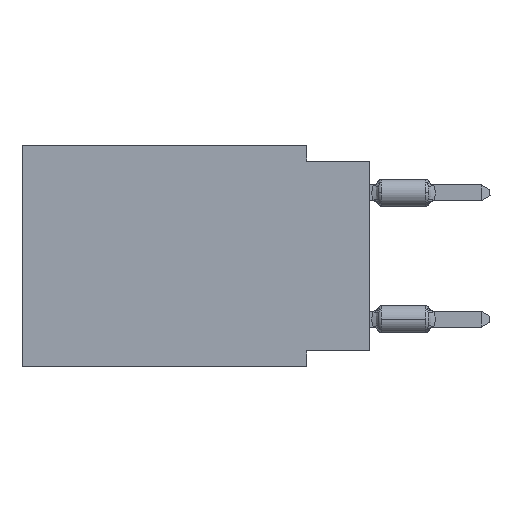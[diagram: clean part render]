
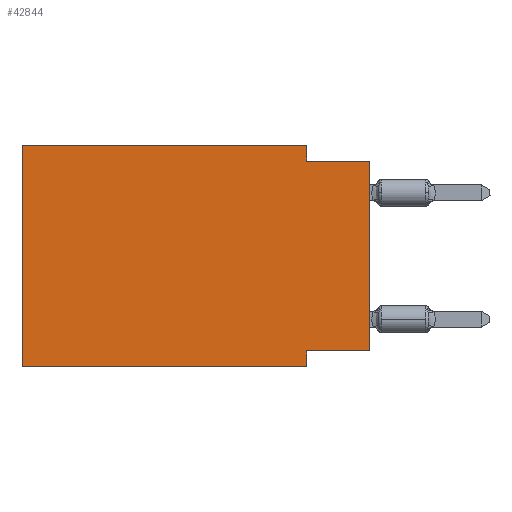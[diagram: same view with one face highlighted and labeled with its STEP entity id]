
A CAD part, left-side view. The second image highlights one B-rep face of the part: STEP entity #42844.
In plain terms, the highlighted planar face has unit normal (-1, 0, 0).
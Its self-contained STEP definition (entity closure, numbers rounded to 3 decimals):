
#47 = LINE ( 'NONE', #48566, #8587 ) ;
#1455 = VERTEX_POINT ( 'NONE', #36097 ) ;
#1940 = EDGE_CURVE ( 'NONE', #30021, #1455, #11986, .T. ) ;
#6177 = VECTOR ( 'NONE', #21115, 1000. ) ;
#7460 = DIRECTION ( 'NONE',  ( 0., 1., 0. ) ) ;
#7759 = ORIENTED_EDGE ( 'NONE', *, *, #32227, .F. ) ;
#8587 = VECTOR ( 'NONE', #56101, 1000. ) ;
#8679 = CARTESIAN_POINT ( 'NONE',  ( 0., 13.97, -8.89 ) ) ;
#11063 = VERTEX_POINT ( 'NONE', #21860 ) ;
#11986 = LINE ( 'NONE', #51801, #17896 ) ;
#12231 = ORIENTED_EDGE ( 'NONE', *, *, #14023, .T. ) ;
#12671 = VERTEX_POINT ( 'NONE', #51534 ) ;
#13455 = DIRECTION ( 'NONE',  ( 1., 0., 0. ) ) ;
#14023 = EDGE_CURVE ( 'NONE', #19045, #12671, #47, .T. ) ;
#15054 = DIRECTION ( 'NONE',  ( 0., 0., -1. ) ) ;
#15900 = DIRECTION ( 'NONE',  ( 0., -1., 0. ) ) ;
#16130 = LINE ( 'NONE', #34026, #16550 ) ;
#16370 = DIRECTION ( 'NONE',  ( 0., -1., 0. ) ) ;
#16550 = VECTOR ( 'NONE', #7460, 1000. ) ;
#16808 = ORIENTED_EDGE ( 'NONE', *, *, #52553, .F. ) ;
#16925 = LINE ( 'NONE', #51840, #30788 ) ;
#17685 = CARTESIAN_POINT ( 'NONE',  ( 0., 2.54, 0. ) ) ;
#17896 = VECTOR ( 'NONE', #34499, 1000. ) ;
#18069 = PLANE ( 'NONE',  #54730 ) ;
#18987 = EDGE_CURVE ( 'NONE', #24893, #30021, #28609, .T. ) ;
#19045 = VERTEX_POINT ( 'NONE', #42176 ) ;
#19066 = VERTEX_POINT ( 'NONE', #28044 ) ;
#19434 = ORIENTED_EDGE ( 'NONE', *, *, #37100, .F. ) ;
#19956 = LINE ( 'NONE', #37571, #31787 ) ;
#20986 = CARTESIAN_POINT ( 'NONE',  ( 0., 0., -0.635 ) ) ;
#21115 = DIRECTION ( 'NONE',  ( 0., -1., 0. ) ) ;
#21860 = CARTESIAN_POINT ( 'NONE',  ( 0., 13.97, -8.89 ) ) ;
#22683 = DIRECTION ( 'NONE',  ( 0., 0., -1. ) ) ;
#23450 = EDGE_LOOP ( 'NONE', ( #12231, #16808, #46729, #43079, #19434, #29233, #45018, #7759 ) ) ;
#24812 = CARTESIAN_POINT ( 'NONE',  ( 0., 13.97, 0. ) ) ;
#24893 = VERTEX_POINT ( 'NONE', #24812 ) ;
#25732 = LINE ( 'NONE', #8679, #6177 ) ;
#28044 = CARTESIAN_POINT ( 'NONE',  ( 0., 2.54, -8.255 ) ) ;
#28609 = LINE ( 'NONE', #55429, #52073 ) ;
#29028 = VERTEX_POINT ( 'NONE', #46916 ) ;
#29233 = ORIENTED_EDGE ( 'NONE', *, *, #50389, .T. ) ;
#30021 = VERTEX_POINT ( 'NONE', #17685 ) ;
#30702 = VECTOR ( 'NONE', #16370, 1000. ) ;
#30788 = VECTOR ( 'NONE', #47242, 1000. ) ;
#31787 = VECTOR ( 'NONE', #15054, 1000. ) ;
#32227 = EDGE_CURVE ( 'NONE', #19045, #19066, #16130, .T. ) ;
#34026 = CARTESIAN_POINT ( 'NONE',  ( 0., 0., -8.255 ) ) ;
#34499 = DIRECTION ( 'NONE',  ( 0., 0., -1. ) ) ;
#36097 = CARTESIAN_POINT ( 'NONE',  ( 0., 2.54, -0.635 ) ) ;
#37100 = EDGE_CURVE ( 'NONE', #11063, #24893, #16925, .T. ) ;
#37571 = CARTESIAN_POINT ( 'NONE',  ( 0., 2.54, -8.89 ) ) ;
#42176 = CARTESIAN_POINT ( 'NONE',  ( 0., 0., -8.255 ) ) ;
#42844 = ADVANCED_FACE ( 'NONE', ( #43498 ), #18069, .F. ) ;
#43079 = ORIENTED_EDGE ( 'NONE', *, *, #18987, .F. ) ;
#43498 = FACE_OUTER_BOUND ( 'NONE', #23450, .T. ) ;
#44333 = CARTESIAN_POINT ( 'NONE',  ( 0., 13.97, 0. ) ) ;
#45018 = ORIENTED_EDGE ( 'NONE', *, *, #57055, .F. ) ;
#46729 = ORIENTED_EDGE ( 'NONE', *, *, #1940, .F. ) ;
#46916 = CARTESIAN_POINT ( 'NONE',  ( 0., 2.54, -8.89 ) ) ;
#47242 = DIRECTION ( 'NONE',  ( 0., 0., 1. ) ) ;
#48566 = CARTESIAN_POINT ( 'NONE',  ( 0., 0., 0. ) ) ;
#50389 = EDGE_CURVE ( 'NONE', #11063, #29028, #25732, .T. ) ;
#51534 = CARTESIAN_POINT ( 'NONE',  ( 0., 0., -0.635 ) ) ;
#51801 = CARTESIAN_POINT ( 'NONE',  ( 0., 2.54, 0. ) ) ;
#51840 = CARTESIAN_POINT ( 'NONE',  ( 0., 13.97, 0. ) ) ;
#52073 = VECTOR ( 'NONE', #15900, 1000. ) ;
#52553 = EDGE_CURVE ( 'NONE', #1455, #12671, #55903, .T. ) ;
#54730 = AXIS2_PLACEMENT_3D ( 'NONE', #44333, #13455, #22683 ) ;
#55429 = CARTESIAN_POINT ( 'NONE',  ( 0., 13.97, 0. ) ) ;
#55903 = LINE ( 'NONE', #20986, #30702 ) ;
#56101 = DIRECTION ( 'NONE',  ( 0., 0., 1. ) ) ;
#57055 = EDGE_CURVE ( 'NONE', #19066, #29028, #19956, .T. ) ;
